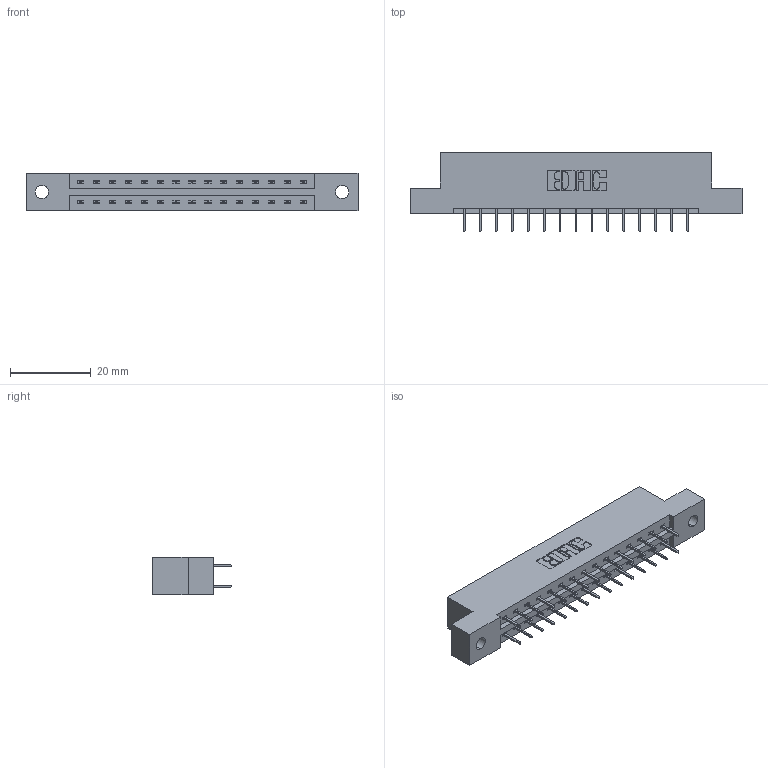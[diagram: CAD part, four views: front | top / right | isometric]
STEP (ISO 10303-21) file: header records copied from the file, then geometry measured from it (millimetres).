
FILE_DESCRIPTION (( 'STEP AP203' ), '1' );
FILE_NAME ('337-030-524-202.STEP', '2018-08-07T00:42:18', ( '' ), ( '' ), 'SwSTEP 2.0', 'SolidWorks 2016', '' );
FILE_SCHEMA (( 'CONFIG_CONTROL_DESIGN' ));
Length unit declared in the file: inch
Products named in the file (3): 337 Part_Flush Mounting Lugs - 0.128 Dia; 345-292-001_345-293-124; 337-030-524-202
Assembly tree (31 placements, depth 2):
  337-030-524-202
    337 Part_Flush Mounting Lugs - 0.128 Dia
    345-292-001_345-293-124  x30
Bounding box: 82.45 x 19.69 x 9.4 mm (x, y, z)
Volume: 8247.6 mm3; surface area: 8648.3 mm2
Topology: 31 solids, 31 shells, 1854 faces, 5261 edges, 3386 vertices
Faces by surface type: plane 1390, cylinder 464
Entity records: 15199 total; most frequent: CARTESIAN_POINT 2582, ORIENTED_EDGE 2518, DIRECTION 2247, EDGE_CURVE 1259, LINE 1135, VECTOR 1135, VERTEX_POINT 834, AXIS2_PLACEMENT_3D 556
